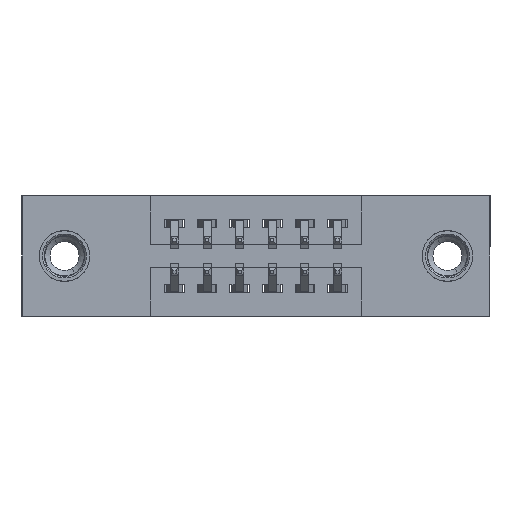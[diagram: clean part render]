
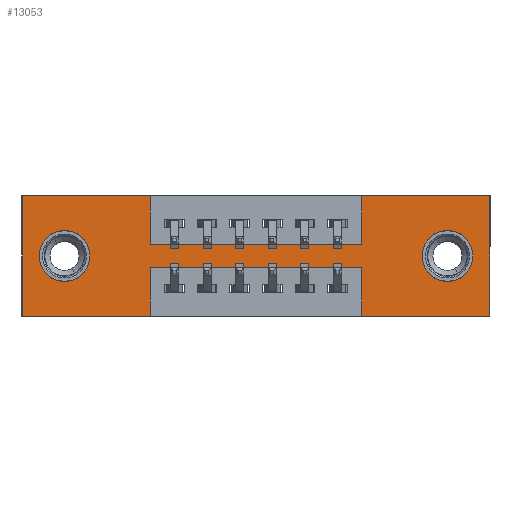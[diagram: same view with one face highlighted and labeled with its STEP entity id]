
A CAD part, front view. The second image highlights one B-rep face of the part: STEP entity #13053.
In plain terms, the highlighted planar face has unit normal (0, -1, 0).
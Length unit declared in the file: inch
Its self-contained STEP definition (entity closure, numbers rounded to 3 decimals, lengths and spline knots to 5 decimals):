
#35 = EDGE_CURVE ( 'NONE', #2212, #10725, #2227, .T. ) ;
#79 = LINE ( 'NONE', #11421, #4264 ) ;
#284 = EDGE_CURVE ( 'NONE', #5577, #2424, #477, .T. ) ;
#323 = DIRECTION ( 'NONE',  ( 0., 0., -1. ) ) ;
#477 = LINE ( 'NONE', #5689, #5692 ) ;
#491 = CARTESIAN_POINT ( 'NONE',  ( 0., 0., -0.37 ) ) ;
#547 = CARTESIAN_POINT ( 'NONE',  ( 1.0425, 0., -0.22 ) ) ;
#555 = DIRECTION ( 'NONE',  ( -1., 0., 0. ) ) ;
#651 = CARTESIAN_POINT ( 'NONE',  ( 0., 0., -0.37 ) ) ;
#704 = VERTEX_POINT ( 'NONE', #9769 ) ;
#812 = CARTESIAN_POINT ( 'NONE',  ( 0., 0., -0.37 ) ) ;
#942 = ORIENTED_EDGE ( 'NONE', *, *, #1060, .F. ) ;
#1053 = EDGE_CURVE ( 'NONE', #13427, #7081, #79, .T. ) ;
#1060 = EDGE_CURVE ( 'NONE', #8148, #5987, #3213, .T. ) ;
#1234 = DIRECTION ( 'NONE',  ( 0., 0., 1. ) ) ;
#1284 = LINE ( 'NONE', #3762, #14317 ) ;
#1409 = EDGE_CURVE ( 'NONE', #3684, #3445, #4232, .T. ) ;
#1548 = DIRECTION ( 'NONE',  ( 0., 0., -1. ) ) ;
#2212 = VERTEX_POINT ( 'NONE', #7522 ) ;
#2227 = LINE ( 'NONE', #9619, #4157 ) ;
#2260 = FACE_BOUND ( 'NONE', #2639, .T. ) ;
#2399 = CIRCLE ( 'NONE', #6619, 0.078 ) ;
#2424 = VERTEX_POINT ( 'NONE', #2509 ) ;
#2508 = CARTESIAN_POINT ( 'NONE',  ( 1.0425, 0., 0. ) ) ;
#2509 = CARTESIAN_POINT ( 'NONE',  ( 0.3925, 0., -0.37 ) ) ;
#2569 = DIRECTION ( 'NONE',  ( -1., 0., 0. ) ) ;
#2639 = EDGE_LOOP ( 'NONE', ( #11383, #14479 ) ) ;
#2846 = EDGE_LOOP ( 'NONE', ( #9507, #5916 ) ) ;
#2866 = CARTESIAN_POINT ( 'NONE',  ( 1.305, 0., -0.263 ) ) ;
#2965 = EDGE_CURVE ( 'NONE', #5987, #2212, #3316, .T. ) ;
#3102 = VERTEX_POINT ( 'NONE', #5825 ) ;
#3213 = LINE ( 'NONE', #2508, #4255 ) ;
#3313 = EDGE_CURVE ( 'NONE', #2424, #9012, #10052, .T. ) ;
#3316 = LINE ( 'NONE', #4272, #5945 ) ;
#3445 = VERTEX_POINT ( 'NONE', #6365 ) ;
#3684 = VERTEX_POINT ( 'NONE', #8714 ) ;
#3762 = CARTESIAN_POINT ( 'NONE',  ( 0.3925, 0., -0.22 ) ) ;
#3829 = EDGE_CURVE ( 'NONE', #10725, #13427, #12504, .T. ) ;
#3988 = ORIENTED_EDGE ( 'NONE', *, *, #3829, .F. ) ;
#4157 = VECTOR ( 'NONE', #4998, 39.37008 ) ;
#4158 = CARTESIAN_POINT ( 'NONE',  ( 0.3925, 0., -0.15 ) ) ;
#4232 = LINE ( 'NONE', #8198, #6495 ) ;
#4255 = VECTOR ( 'NONE', #9151, 39.37008 ) ;
#4264 = VECTOR ( 'NONE', #9297, 39.37008 ) ;
#4272 = CARTESIAN_POINT ( 'NONE',  ( 0., 0., 0. ) ) ;
#4425 = DIRECTION ( 'NONE',  ( 0., 1., 0. ) ) ;
#4439 = DIRECTION ( 'NONE',  ( 0., -1., 0. ) ) ;
#4602 = ORIENTED_EDGE ( 'NONE', *, *, #1409, .F. ) ;
#4722 = AXIS2_PLACEMENT_3D ( 'NONE', #812, #4439, #6723 ) ;
#4757 = DIRECTION ( 'NONE',  ( 0., 0., -1. ) ) ;
#4768 = CARTESIAN_POINT ( 'NONE',  ( 0., 0., -0.37 ) ) ;
#4806 = EDGE_LOOP ( 'NONE', ( #14373, #7504, #10247, #3988, #10850, #11528, #942, #14427, #4602, #5979, #13046, #6177 ) ) ;
#4998 = DIRECTION ( 'NONE',  ( 0., 0., -1. ) ) ;
#5501 = VERTEX_POINT ( 'NONE', #6777 ) ;
#5577 = VERTEX_POINT ( 'NONE', #14141 ) ;
#5689 = CARTESIAN_POINT ( 'NONE',  ( 0.3925, 0., -0.37 ) ) ;
#5692 = VECTOR ( 'NONE', #323, 39.37008 ) ;
#5763 = DIRECTION ( 'NONE',  ( 0., 1., 0. ) ) ;
#5825 = CARTESIAN_POINT ( 'NONE',  ( 0.13, 0., -0.263 ) ) ;
#5879 = CARTESIAN_POINT ( 'NONE',  ( 1.0425, 0., -0.37 ) ) ;
#5916 = ORIENTED_EDGE ( 'NONE', *, *, #12809, .T. ) ;
#5945 = VECTOR ( 'NONE', #10879, 39.37008 ) ;
#5979 = ORIENTED_EDGE ( 'NONE', *, *, #8138, .F. ) ;
#5987 = VERTEX_POINT ( 'NONE', #10279 ) ;
#5999 = DIRECTION ( 'NONE',  ( 0., 0., -1. ) ) ;
#6007 = VECTOR ( 'NONE', #2569, 39.37008 ) ;
#6100 = CARTESIAN_POINT ( 'NONE',  ( 1.435, 0., -0.37 ) ) ;
#6177 = ORIENTED_EDGE ( 'NONE', *, *, #3313, .F. ) ;
#6274 = AXIS2_PLACEMENT_3D ( 'NONE', #9079, #5763, #13590 ) ;
#6365 = CARTESIAN_POINT ( 'NONE',  ( 0.3925, 0., -0.15 ) ) ;
#6459 = EDGE_CURVE ( 'NONE', #3445, #8148, #8387, .T. ) ;
#6495 = VECTOR ( 'NONE', #4757, 39.37008 ) ;
#6619 = AXIS2_PLACEMENT_3D ( 'NONE', #7943, #4425, #1234 ) ;
#6666 = VECTOR ( 'NONE', #555, 39.37008 ) ;
#6723 = DIRECTION ( 'NONE',  ( 0., 0., -1. ) ) ;
#6744 = VECTOR ( 'NONE', #10591, 39.37008 ) ;
#6777 = CARTESIAN_POINT ( 'NONE',  ( 1.305, 0., -0.107 ) ) ;
#6923 = EDGE_CURVE ( 'NONE', #9716, #3102, #8736, .T. ) ;
#6931 = CIRCLE ( 'NONE', #12780, 0.078 ) ;
#7081 = VERTEX_POINT ( 'NONE', #547 ) ;
#7158 = DIRECTION ( 'NONE',  ( 0., 1., 0. ) ) ;
#7263 = DIRECTION ( 'NONE',  ( 0., 1., 0. ) ) ;
#7504 = ORIENTED_EDGE ( 'NONE', *, *, #9102, .F. ) ;
#7522 = CARTESIAN_POINT ( 'NONE',  ( 1.435, 0., 0. ) ) ;
#7807 = EDGE_CURVE ( 'NONE', #5501, #7919, #6931, .T. ) ;
#7919 = VERTEX_POINT ( 'NONE', #2866 ) ;
#7943 = CARTESIAN_POINT ( 'NONE',  ( 0.13, 0., -0.185 ) ) ;
#8027 = FACE_BOUND ( 'NONE', #2846, .T. ) ;
#8138 = EDGE_CURVE ( 'NONE', #704, #3684, #11177, .T. ) ;
#8148 = VERTEX_POINT ( 'NONE', #10635 ) ;
#8198 = CARTESIAN_POINT ( 'NONE',  ( 0.3925, 0., 0. ) ) ;
#8387 = LINE ( 'NONE', #4158, #14241 ) ;
#8714 = CARTESIAN_POINT ( 'NONE',  ( 0.3925, 0., 0. ) ) ;
#8736 = CIRCLE ( 'NONE', #6274, 0.078 ) ;
#9012 = VERTEX_POINT ( 'NONE', #491 ) ;
#9074 = AXIS2_PLACEMENT_3D ( 'NONE', #11511, #7158, #5999 ) ;
#9079 = CARTESIAN_POINT ( 'NONE',  ( 0.13, 0., -0.185 ) ) ;
#9102 = EDGE_CURVE ( 'NONE', #7081, #5577, #1284, .T. ) ;
#9151 = DIRECTION ( 'NONE',  ( 0., 0., 1. ) ) ;
#9297 = DIRECTION ( 'NONE',  ( 0., 0., 1. ) ) ;
#9477 = CIRCLE ( 'NONE', #9074, 0.078 ) ;
#9507 = ORIENTED_EDGE ( 'NONE', *, *, #7807, .T. ) ;
#9619 = CARTESIAN_POINT ( 'NONE',  ( 1.435, 0., 0. ) ) ;
#9716 = VERTEX_POINT ( 'NONE', #14318 ) ;
#9769 = CARTESIAN_POINT ( 'NONE',  ( 0., 0., 0. ) ) ;
#9928 = DIRECTION ( 'NONE',  ( -1., 0., 0. ) ) ;
#10023 = DIRECTION ( 'NONE',  ( 1., 0., 0. ) ) ;
#10052 = LINE ( 'NONE', #651, #6666 ) ;
#10247 = ORIENTED_EDGE ( 'NONE', *, *, #1053, .F. ) ;
#10279 = CARTESIAN_POINT ( 'NONE',  ( 1.0425, 0., 0. ) ) ;
#10319 = EDGE_CURVE ( 'NONE', #9012, #704, #13736, .T. ) ;
#10591 = DIRECTION ( 'NONE',  ( 1., 0., 0. ) ) ;
#10635 = CARTESIAN_POINT ( 'NONE',  ( 1.0425, 0., -0.15 ) ) ;
#10725 = VERTEX_POINT ( 'NONE', #6100 ) ;
#10850 = ORIENTED_EDGE ( 'NONE', *, *, #35, .F. ) ;
#10879 = DIRECTION ( 'NONE',  ( 1., 0., 0. ) ) ;
#11177 = LINE ( 'NONE', #11912, #6744 ) ;
#11383 = ORIENTED_EDGE ( 'NONE', *, *, #6923, .T. ) ;
#11421 = CARTESIAN_POINT ( 'NONE',  ( 1.0425, 0., -0.37 ) ) ;
#11511 = CARTESIAN_POINT ( 'NONE',  ( 1.305, 0., -0.185 ) ) ;
#11528 = ORIENTED_EDGE ( 'NONE', *, *, #2965, .F. ) ;
#11912 = CARTESIAN_POINT ( 'NONE',  ( 0., 0., 0. ) ) ;
#11938 = CARTESIAN_POINT ( 'NONE',  ( 0., 0., 0. ) ) ;
#12401 = DIRECTION ( 'NONE',  ( 0., 0., 1. ) ) ;
#12504 = LINE ( 'NONE', #4768, #6007 ) ;
#12780 = AXIS2_PLACEMENT_3D ( 'NONE', #14034, #7263, #1548 ) ;
#12809 = EDGE_CURVE ( 'NONE', #7919, #5501, #9477, .T. ) ;
#13046 = ORIENTED_EDGE ( 'NONE', *, *, #10319, .F. ) ;
#13053 = ADVANCED_FACE ( 'NONE', ( #8027, #2260, #13873 ), #14286, .T. ) ;
#13427 = VERTEX_POINT ( 'NONE', #5879 ) ;
#13590 = DIRECTION ( 'NONE',  ( 0., 0., 1. ) ) ;
#13720 = EDGE_CURVE ( 'NONE', #3102, #9716, #2399, .T. ) ;
#13736 = LINE ( 'NONE', #11938, #13930 ) ;
#13873 = FACE_OUTER_BOUND ( 'NONE', #4806, .T. ) ;
#13930 = VECTOR ( 'NONE', #12401, 39.37008 ) ;
#14034 = CARTESIAN_POINT ( 'NONE',  ( 1.305, 0., -0.185 ) ) ;
#14141 = CARTESIAN_POINT ( 'NONE',  ( 0.3925, 0., -0.22 ) ) ;
#14241 = VECTOR ( 'NONE', #10023, 39.37008 ) ;
#14286 = PLANE ( 'NONE',  #4722 ) ;
#14317 = VECTOR ( 'NONE', #9928, 39.37008 ) ;
#14318 = CARTESIAN_POINT ( 'NONE',  ( 0.13, 0., -0.107 ) ) ;
#14373 = ORIENTED_EDGE ( 'NONE', *, *, #284, .F. ) ;
#14427 = ORIENTED_EDGE ( 'NONE', *, *, #6459, .F. ) ;
#14479 = ORIENTED_EDGE ( 'NONE', *, *, #13720, .T. ) ;
